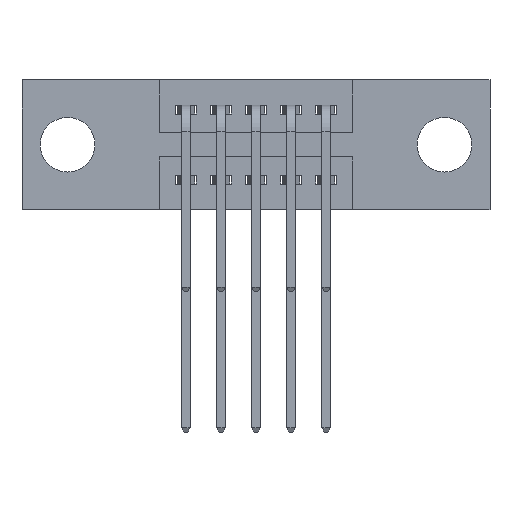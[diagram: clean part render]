
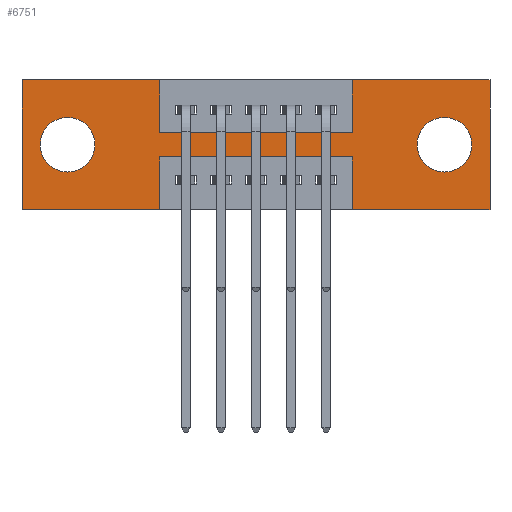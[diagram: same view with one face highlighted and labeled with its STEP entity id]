
A CAD part, front view. The second image highlights one B-rep face of the part: STEP entity #6751.
In plain terms, the highlighted planar face has unit normal (0, -1, 0).
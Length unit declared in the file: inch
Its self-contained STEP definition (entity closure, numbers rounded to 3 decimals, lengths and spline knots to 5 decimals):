
#142 = CARTESIAN_POINT ( 'NONE',  ( 0.9425, 0., -0.37 ) ) ;
#177 = DIRECTION ( 'NONE',  ( 0., -1., 0. ) ) ;
#216 = LINE ( 'NONE', #841, #10097 ) ;
#251 = EDGE_CURVE ( 'NONE', #8215, #926, #9457, .T. ) ;
#451 = CARTESIAN_POINT ( 'NONE',  ( 0.13, 0., -0.263 ) ) ;
#509 = CARTESIAN_POINT ( 'NONE',  ( 0., 0., 0. ) ) ;
#518 = CARTESIAN_POINT ( 'NONE',  ( 0., 0., -0.37 ) ) ;
#523 = CARTESIAN_POINT ( 'NONE',  ( 0.9425, 0., -0.22 ) ) ;
#753 = EDGE_CURVE ( 'NONE', #10322, #2114, #798, .T. ) ;
#798 = LINE ( 'NONE', #4194, #4500 ) ;
#841 = CARTESIAN_POINT ( 'NONE',  ( 0.3925, 0., 0. ) ) ;
#926 = VERTEX_POINT ( 'NONE', #8554 ) ;
#954 = DIRECTION ( 'NONE',  ( 0., 1., 0. ) ) ;
#959 = DIRECTION ( 'NONE',  ( 0., 0., -1. ) ) ;
#973 = DIRECTION ( 'NONE',  ( 0., 0., -1. ) ) ;
#1036 = EDGE_LOOP ( 'NONE', ( #1652, #5893 ) ) ;
#1049 = ORIENTED_EDGE ( 'NONE', *, *, #8003, .F. ) ;
#1068 = DIRECTION ( 'NONE',  ( 0., 0., 1. ) ) ;
#1323 = CIRCLE ( 'NONE', #2939, 0.078 ) ;
#1350 = ORIENTED_EDGE ( 'NONE', *, *, #9842, .F. ) ;
#1355 = CARTESIAN_POINT ( 'NONE',  ( 0.3925, 0., -0.15 ) ) ;
#1452 = CARTESIAN_POINT ( 'NONE',  ( 0.9425, 0., 0. ) ) ;
#1627 = EDGE_CURVE ( 'NONE', #7705, #10243, #3190, .T. ) ;
#1651 = ORIENTED_EDGE ( 'NONE', *, *, #753, .F. ) ;
#1652 = ORIENTED_EDGE ( 'NONE', *, *, #9075, .T. ) ;
#1735 = FACE_BOUND ( 'NONE', #5157, .T. ) ;
#1832 = VERTEX_POINT ( 'NONE', #7163 ) ;
#1912 = VECTOR ( 'NONE', #7827, 39.37008 ) ;
#2015 = LINE ( 'NONE', #10674, #3535 ) ;
#2023 = VECTOR ( 'NONE', #4797, 39.37008 ) ;
#2085 = ORIENTED_EDGE ( 'NONE', *, *, #1627, .F. ) ;
#2114 = VERTEX_POINT ( 'NONE', #10379 ) ;
#2203 = DIRECTION ( 'NONE',  ( 1., 0., 0. ) ) ;
#2243 = CARTESIAN_POINT ( 'NONE',  ( 1.205, 0., -0.107 ) ) ;
#2433 = ORIENTED_EDGE ( 'NONE', *, *, #8188, .F. ) ;
#2511 = CARTESIAN_POINT ( 'NONE',  ( 0.3925, 0., -0.37 ) ) ;
#2527 = VERTEX_POINT ( 'NONE', #8246 ) ;
#2560 = CARTESIAN_POINT ( 'NONE',  ( 0., 0., 0. ) ) ;
#2568 = CARTESIAN_POINT ( 'NONE',  ( 0.13, 0., -0.185 ) ) ;
#2728 = VERTEX_POINT ( 'NONE', #10483 ) ;
#2735 = CARTESIAN_POINT ( 'NONE',  ( 0., 0., -0.37 ) ) ;
#2939 = AXIS2_PLACEMENT_3D ( 'NONE', #4736, #3754, #7967 ) ;
#2981 = CARTESIAN_POINT ( 'NONE',  ( 0., 0., -0.37 ) ) ;
#3117 = LINE ( 'NONE', #509, #5458 ) ;
#3165 = VECTOR ( 'NONE', #1068, 39.37008 ) ;
#3190 = LINE ( 'NONE', #518, #2023 ) ;
#3232 = DIRECTION ( 'NONE',  ( 0., 0., -1. ) ) ;
#3309 = VECTOR ( 'NONE', #10961, 39.37008 ) ;
#3351 = DIRECTION ( 'NONE',  ( 0., 0., -1. ) ) ;
#3403 = LINE ( 'NONE', #2560, #10911 ) ;
#3535 = VECTOR ( 'NONE', #5404, 39.37008 ) ;
#3596 = CARTESIAN_POINT ( 'NONE',  ( 1.335, 0., 0. ) ) ;
#3603 = AXIS2_PLACEMENT_3D ( 'NONE', #2568, #954, #4297 ) ;
#3654 = CARTESIAN_POINT ( 'NONE',  ( 0.3925, 0., -0.37 ) ) ;
#3754 = DIRECTION ( 'NONE',  ( 0., 1., 0. ) ) ;
#3909 = DIRECTION ( 'NONE',  ( 1., 0., 0. ) ) ;
#4147 = EDGE_CURVE ( 'NONE', #7528, #10322, #10639, .T. ) ;
#4150 = VERTEX_POINT ( 'NONE', #2243 ) ;
#4194 = CARTESIAN_POINT ( 'NONE',  ( 0., 0., 0. ) ) ;
#4250 = PLANE ( 'NONE',  #10946 ) ;
#4297 = DIRECTION ( 'NONE',  ( 0., 0., 1. ) ) ;
#4484 = EDGE_CURVE ( 'NONE', #926, #8215, #1323, .T. ) ;
#4500 = VECTOR ( 'NONE', #8356, 39.37008 ) ;
#4539 = ORIENTED_EDGE ( 'NONE', *, *, #9725, .F. ) ;
#4575 = CIRCLE ( 'NONE', #10771, 0.078 ) ;
#4736 = CARTESIAN_POINT ( 'NONE',  ( 0.13, 0., -0.185 ) ) ;
#4797 = DIRECTION ( 'NONE',  ( -1., 0., 0. ) ) ;
#4800 = EDGE_CURVE ( 'NONE', #10400, #8149, #3403, .T. ) ;
#4811 = CARTESIAN_POINT ( 'NONE',  ( 1.205, 0., -0.185 ) ) ;
#5063 = ORIENTED_EDGE ( 'NONE', *, *, #251, .T. ) ;
#5135 = FACE_OUTER_BOUND ( 'NONE', #10466, .T. ) ;
#5157 = EDGE_LOOP ( 'NONE', ( #6878, #5063 ) ) ;
#5235 = ORIENTED_EDGE ( 'NONE', *, *, #10928, .F. ) ;
#5288 = DIRECTION ( 'NONE',  ( 0., 0., -1. ) ) ;
#5404 = DIRECTION ( 'NONE',  ( 0., 0., 1. ) ) ;
#5458 = VECTOR ( 'NONE', #3909, 39.37008 ) ;
#5490 = AXIS2_PLACEMENT_3D ( 'NONE', #4811, #7415, #9140 ) ;
#5520 = CARTESIAN_POINT ( 'NONE',  ( 0.3925, 0., -0.15 ) ) ;
#5627 = CARTESIAN_POINT ( 'NONE',  ( 0., 0., -0.37 ) ) ;
#5879 = DIRECTION ( 'NONE',  ( 1., 0., 0. ) ) ;
#5893 = ORIENTED_EDGE ( 'NONE', *, *, #10897, .T. ) ;
#6258 = CARTESIAN_POINT ( 'NONE',  ( 0.3925, 0., -0.22 ) ) ;
#6361 = EDGE_CURVE ( 'NONE', #8149, #7705, #6805, .T. ) ;
#6388 = CARTESIAN_POINT ( 'NONE',  ( 1.335, 0., 0. ) ) ;
#6451 = CARTESIAN_POINT ( 'NONE',  ( 1.335, 0., -0.37 ) ) ;
#6468 = VERTEX_POINT ( 'NONE', #5520 ) ;
#6485 = VERTEX_POINT ( 'NONE', #523 ) ;
#6516 = VECTOR ( 'NONE', #2203, 39.37008 ) ;
#6751 = ADVANCED_FACE ( 'NONE', ( #9360, #1735, #5135 ), #4250, .T. ) ;
#6805 = LINE ( 'NONE', #3596, #9358 ) ;
#6878 = ORIENTED_EDGE ( 'NONE', *, *, #4484, .T. ) ;
#6891 = VERTEX_POINT ( 'NONE', #7177 ) ;
#6990 = EDGE_CURVE ( 'NONE', #2114, #6891, #3117, .T. ) ;
#7163 = CARTESIAN_POINT ( 'NONE',  ( 0.3925, 0., -0.22 ) ) ;
#7177 = CARTESIAN_POINT ( 'NONE',  ( 0.3925, 0., 0. ) ) ;
#7309 = LINE ( 'NONE', #1355, #6516 ) ;
#7395 = DIRECTION ( 'NONE',  ( 0., 1., 0. ) ) ;
#7415 = DIRECTION ( 'NONE',  ( 0., 1., 0. ) ) ;
#7528 = VERTEX_POINT ( 'NONE', #3654 ) ;
#7556 = CARTESIAN_POINT ( 'NONE',  ( 1.205, 0., -0.185 ) ) ;
#7638 = ORIENTED_EDGE ( 'NONE', *, *, #4800, .F. ) ;
#7705 = VERTEX_POINT ( 'NONE', #6451 ) ;
#7827 = DIRECTION ( 'NONE',  ( -1., 0., 0. ) ) ;
#7967 = DIRECTION ( 'NONE',  ( 0., 0., 1. ) ) ;
#8003 = EDGE_CURVE ( 'NONE', #2527, #10400, #10303, .T. ) ;
#8149 = VERTEX_POINT ( 'NONE', #6388 ) ;
#8188 = EDGE_CURVE ( 'NONE', #10243, #6485, #2015, .T. ) ;
#8215 = VERTEX_POINT ( 'NONE', #451 ) ;
#8246 = CARTESIAN_POINT ( 'NONE',  ( 0.9425, 0., -0.15 ) ) ;
#8356 = DIRECTION ( 'NONE',  ( 0., 0., 1. ) ) ;
#8422 = EDGE_CURVE ( 'NONE', #6891, #6468, #216, .T. ) ;
#8554 = CARTESIAN_POINT ( 'NONE',  ( 0.13, 0., -0.107 ) ) ;
#9041 = CIRCLE ( 'NONE', #5490, 0.078 ) ;
#9075 = EDGE_CURVE ( 'NONE', #4150, #2728, #9041, .T. ) ;
#9140 = DIRECTION ( 'NONE',  ( 0., 0., -1. ) ) ;
#9171 = ORIENTED_EDGE ( 'NONE', *, *, #6361, .F. ) ;
#9179 = LINE ( 'NONE', #2511, #10604 ) ;
#9205 = ORIENTED_EDGE ( 'NONE', *, *, #4147, .F. ) ;
#9358 = VECTOR ( 'NONE', #973, 39.37008 ) ;
#9360 = FACE_BOUND ( 'NONE', #1036, .T. ) ;
#9457 = CIRCLE ( 'NONE', #3603, 0.078 ) ;
#9725 = EDGE_CURVE ( 'NONE', #6485, #1832, #10383, .T. ) ;
#9743 = ORIENTED_EDGE ( 'NONE', *, *, #8422, .F. ) ;
#9842 = EDGE_CURVE ( 'NONE', #6468, #2527, #7309, .T. ) ;
#10097 = VECTOR ( 'NONE', #5288, 39.37008 ) ;
#10183 = CARTESIAN_POINT ( 'NONE',  ( 0.9425, 0., 0. ) ) ;
#10243 = VERTEX_POINT ( 'NONE', #142 ) ;
#10303 = LINE ( 'NONE', #10183, #3165 ) ;
#10322 = VERTEX_POINT ( 'NONE', #2981 ) ;
#10379 = CARTESIAN_POINT ( 'NONE',  ( 0., 0., 0. ) ) ;
#10383 = LINE ( 'NONE', #6258, #1912 ) ;
#10400 = VERTEX_POINT ( 'NONE', #1452 ) ;
#10403 = ORIENTED_EDGE ( 'NONE', *, *, #6990, .F. ) ;
#10466 = EDGE_LOOP ( 'NONE', ( #5235, #4539, #2433, #2085, #9171, #7638, #1049, #1350, #9743, #10403, #1651, #9205 ) ) ;
#10483 = CARTESIAN_POINT ( 'NONE',  ( 1.205, 0., -0.263 ) ) ;
#10604 = VECTOR ( 'NONE', #3351, 39.37008 ) ;
#10639 = LINE ( 'NONE', #5627, #3309 ) ;
#10674 = CARTESIAN_POINT ( 'NONE',  ( 0.9425, 0., -0.37 ) ) ;
#10771 = AXIS2_PLACEMENT_3D ( 'NONE', #7556, #7395, #3232 ) ;
#10897 = EDGE_CURVE ( 'NONE', #2728, #4150, #4575, .T. ) ;
#10911 = VECTOR ( 'NONE', #5879, 39.37008 ) ;
#10928 = EDGE_CURVE ( 'NONE', #1832, #7528, #9179, .T. ) ;
#10946 = AXIS2_PLACEMENT_3D ( 'NONE', #2735, #177, #959 ) ;
#10961 = DIRECTION ( 'NONE',  ( -1., 0., 0. ) ) ;
